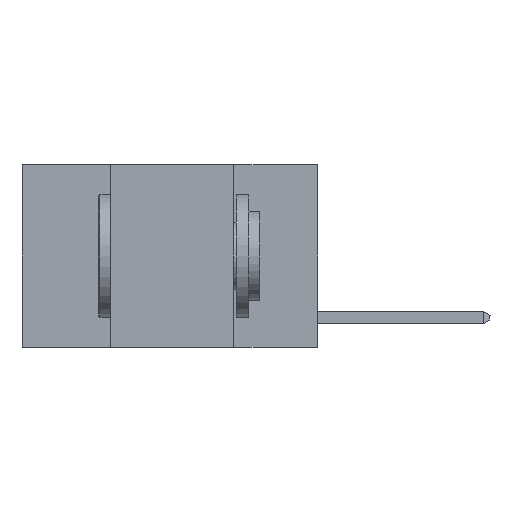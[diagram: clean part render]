
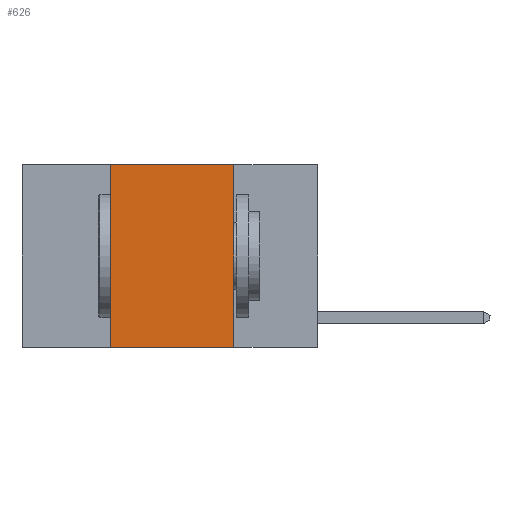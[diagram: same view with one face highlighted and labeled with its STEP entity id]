
A CAD part, left-side view. The second image highlights one B-rep face of the part: STEP entity #626.
In plain terms, the highlighted planar face has unit normal (-1, 0, 0).
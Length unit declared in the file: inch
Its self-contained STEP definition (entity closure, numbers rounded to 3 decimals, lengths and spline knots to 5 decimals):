
#227 = AXIS2_PLACEMENT_3D ( 'NONE', #8013, #19491, #11610 ) ;
#626 = ADVANCED_FACE ( 'NONE', ( #8248 ), #15580, .F. ) ;
#2159 = LINE ( 'NONE', #18530, #14754 ) ;
#2720 = EDGE_CURVE ( 'NONE', #18782, #23705, #14073, .T. ) ;
#3301 = ORIENTED_EDGE ( 'NONE', *, *, #2720, .F. ) ;
#4177 = CARTESIAN_POINT ( 'NONE',  ( 0., 0.42, 0. ) ) ;
#4716 = ORIENTED_EDGE ( 'NONE', *, *, #6027, .F. ) ;
#4747 = VERTEX_POINT ( 'NONE', #18904 ) ;
#5935 = ORIENTED_EDGE ( 'NONE', *, *, #14251, .F. ) ;
#6027 = EDGE_CURVE ( 'NONE', #4747, #11743, #22329, .T. ) ;
#6622 = DIRECTION ( 'NONE',  ( 0., -1., 0. ) ) ;
#8013 = CARTESIAN_POINT ( 'NONE',  ( 0., 0.6, 0. ) ) ;
#8248 = FACE_OUTER_BOUND ( 'NONE', #21980, .T. ) ;
#10810 = DIRECTION ( 'NONE',  ( 0., 0., -1. ) ) ;
#11610 = DIRECTION ( 'NONE',  ( 0., 0., -1. ) ) ;
#11743 = VERTEX_POINT ( 'NONE', #14451 ) ;
#11933 = VECTOR ( 'NONE', #10810, 39.37008 ) ;
#12357 = CARTESIAN_POINT ( 'NONE',  ( 0., 0.17, -0.37 ) ) ;
#13227 = DIRECTION ( 'NONE',  ( 0., 0., 1. ) ) ;
#14073 = LINE ( 'NONE', #14441, #11933 ) ;
#14251 = EDGE_CURVE ( 'NONE', #11743, #18782, #2159, .T. ) ;
#14441 = CARTESIAN_POINT ( 'NONE',  ( 0., 0.17, 0. ) ) ;
#14451 = CARTESIAN_POINT ( 'NONE',  ( 0., 0.42, 0. ) ) ;
#14682 = VECTOR ( 'NONE', #13227, 39.37008 ) ;
#14754 = VECTOR ( 'NONE', #20346, 39.37008 ) ;
#15429 = VECTOR ( 'NONE', #6622, 39.37008 ) ;
#15534 = LINE ( 'NONE', #19321, #15429 ) ;
#15580 = PLANE ( 'NONE',  #227 ) ;
#16598 = ORIENTED_EDGE ( 'NONE', *, *, #16653, .T. ) ;
#16653 = EDGE_CURVE ( 'NONE', #4747, #23705, #15534, .T. ) ;
#18530 = CARTESIAN_POINT ( 'NONE',  ( 0., 0.6, 0. ) ) ;
#18782 = VERTEX_POINT ( 'NONE', #22065 ) ;
#18904 = CARTESIAN_POINT ( 'NONE',  ( 0., 0.42, -0.37 ) ) ;
#19321 = CARTESIAN_POINT ( 'NONE',  ( 0., 0.6, -0.37 ) ) ;
#19491 = DIRECTION ( 'NONE',  ( 1., 0., 0. ) ) ;
#20346 = DIRECTION ( 'NONE',  ( 0., -1., 0. ) ) ;
#21980 = EDGE_LOOP ( 'NONE', ( #3301, #5935, #4716, #16598 ) ) ;
#22065 = CARTESIAN_POINT ( 'NONE',  ( 0., 0.17, 0. ) ) ;
#22329 = LINE ( 'NONE', #4177, #14682 ) ;
#23705 = VERTEX_POINT ( 'NONE', #12357 ) ;
